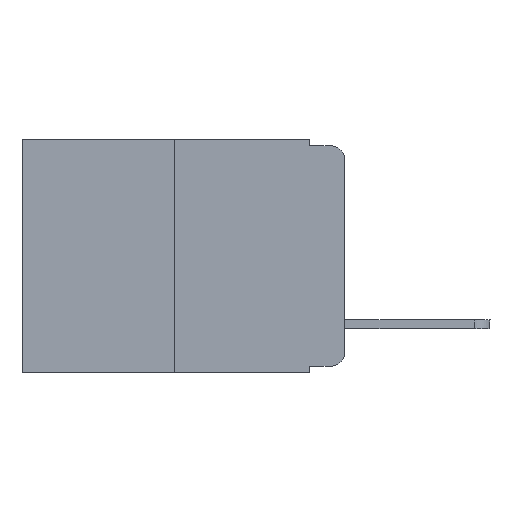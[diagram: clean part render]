
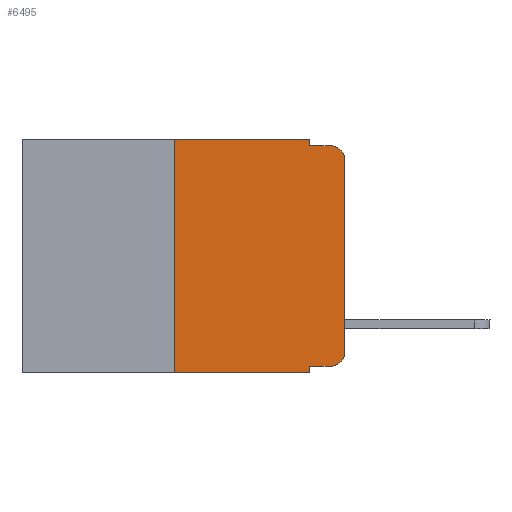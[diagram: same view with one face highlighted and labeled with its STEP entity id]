
A CAD part, left-side view. The second image highlights one B-rep face of the part: STEP entity #6495.
In plain terms, the highlighted planar face has unit normal (-1, 0, 0).
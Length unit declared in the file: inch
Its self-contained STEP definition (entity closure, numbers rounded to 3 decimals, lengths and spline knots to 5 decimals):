
#187 = AXIS2_PLACEMENT_3D ( 'NONE', #8793, #5177, #2572 ) ;
#358 = LINE ( 'NONE', #3914, #7041 ) ;
#514 = VECTOR ( 'NONE', #11091, 39.37008 ) ;
#615 = CARTESIAN_POINT ( 'NONE',  ( 0., 0.051, -0.333 ) ) ;
#802 = CARTESIAN_POINT ( 'NONE',  ( 0., 0.02, -0.01 ) ) ;
#941 = VECTOR ( 'NONE', #5266, 39.37008 ) ;
#1002 = CARTESIAN_POINT ( 'NONE',  ( 0., 0.473, -0.343 ) ) ;
#1118 = LINE ( 'NONE', #1002, #8126 ) ;
#1142 = VERTEX_POINT ( 'NONE', #10294 ) ;
#1150 = CIRCLE ( 'NONE', #4864, 0.02 ) ;
#1329 = FACE_OUTER_BOUND ( 'NONE', #9401, .T. ) ;
#1379 = CARTESIAN_POINT ( 'NONE',  ( 0., 0.02, -0.313 ) ) ;
#1522 = VERTEX_POINT ( 'NONE', #4796 ) ;
#1775 = CARTESIAN_POINT ( 'NONE',  ( 0., 0.25, 0. ) ) ;
#2172 = VECTOR ( 'NONE', #7994, 39.37008 ) ;
#2470 = ORIENTED_EDGE ( 'NONE', *, *, #10821, .F. ) ;
#2572 = DIRECTION ( 'NONE',  ( 0., 0., -1. ) ) ;
#2610 = CARTESIAN_POINT ( 'NONE',  ( 0., 0.473, 0. ) ) ;
#2614 = EDGE_CURVE ( 'NONE', #10281, #10772, #10643, .T. ) ;
#2779 = VECTOR ( 'NONE', #10279, 39.37008 ) ;
#2818 = DIRECTION ( 'NONE',  ( 0., -1., 0. ) ) ;
#2847 = VERTEX_POINT ( 'NONE', #8416 ) ;
#2932 = EDGE_CURVE ( 'NONE', #11075, #1522, #4972, .T. ) ;
#3179 = CARTESIAN_POINT ( 'NONE',  ( 0., 0.051, 0. ) ) ;
#3510 = ORIENTED_EDGE ( 'NONE', *, *, #5780, .T. ) ;
#3914 = CARTESIAN_POINT ( 'NONE',  ( 0., 0.25, 0. ) ) ;
#4440 = CARTESIAN_POINT ( 'NONE',  ( 0., 0.051, 0. ) ) ;
#4601 = ORIENTED_EDGE ( 'NONE', *, *, #9011, .T. ) ;
#4796 = CARTESIAN_POINT ( 'NONE',  ( 0., 0.02, -0.333 ) ) ;
#4849 = VERTEX_POINT ( 'NONE', #5217 ) ;
#4864 = AXIS2_PLACEMENT_3D ( 'NONE', #1379, #6551, #11170 ) ;
#4945 = AXIS2_PLACEMENT_3D ( 'NONE', #5795, #9243, #5850 ) ;
#4972 = LINE ( 'NONE', #615, #2779 ) ;
#4986 = CIRCLE ( 'NONE', #187, 0.02 ) ;
#5103 = CARTESIAN_POINT ( 'NONE',  ( 0., 0., 0. ) ) ;
#5177 = DIRECTION ( 'NONE',  ( -1., 0., 0. ) ) ;
#5215 = EDGE_CURVE ( 'NONE', #1522, #4849, #1150, .T. ) ;
#5217 = CARTESIAN_POINT ( 'NONE',  ( 0., 0., -0.313 ) ) ;
#5266 = DIRECTION ( 'NONE',  ( 0., -1., 0. ) ) ;
#5332 = DIRECTION ( 'NONE',  ( 0., 0., 1. ) ) ;
#5400 = CARTESIAN_POINT ( 'NONE',  ( 0., 0.051, -0.01 ) ) ;
#5403 = ORIENTED_EDGE ( 'NONE', *, *, #7142, .F. ) ;
#5424 = LINE ( 'NONE', #4440, #2172 ) ;
#5591 = DIRECTION ( 'NONE',  ( 0., -1., 0. ) ) ;
#5780 = EDGE_CURVE ( 'NONE', #1142, #8042, #4986, .T. ) ;
#5795 = CARTESIAN_POINT ( 'NONE',  ( 0., 0.473, 0. ) ) ;
#5850 = DIRECTION ( 'NONE',  ( 0., 0., -1. ) ) ;
#6495 = ADVANCED_FACE ( 'NONE', ( #1329 ), #6503, .F. ) ;
#6503 = PLANE ( 'NONE',  #4945 ) ;
#6551 = DIRECTION ( 'NONE',  ( -1., 0., 0. ) ) ;
#6909 = LINE ( 'NONE', #5103, #9968 ) ;
#7041 = VECTOR ( 'NONE', #7451, 39.37008 ) ;
#7142 = EDGE_CURVE ( 'NONE', #11075, #2847, #5424, .T. ) ;
#7417 = LINE ( 'NONE', #3179, #514 ) ;
#7451 = DIRECTION ( 'NONE',  ( 0., 0., 1. ) ) ;
#7865 = ORIENTED_EDGE ( 'NONE', *, *, #8797, .F. ) ;
#7994 = DIRECTION ( 'NONE',  ( 0., 0., -1. ) ) ;
#8042 = VERTEX_POINT ( 'NONE', #802 ) ;
#8126 = VECTOR ( 'NONE', #2818, 39.37008 ) ;
#8128 = EDGE_CURVE ( 'NONE', #4849, #1142, #6909, .T. ) ;
#8416 = CARTESIAN_POINT ( 'NONE',  ( 0., 0.051, -0.343 ) ) ;
#8437 = CARTESIAN_POINT ( 'NONE',  ( 0., 0.051, -0.01 ) ) ;
#8720 = VECTOR ( 'NONE', #5591, 39.37008 ) ;
#8756 = CARTESIAN_POINT ( 'NONE',  ( 0., 0.25, -0.343 ) ) ;
#8793 = CARTESIAN_POINT ( 'NONE',  ( 0., 0.02, -0.03 ) ) ;
#8797 = EDGE_CURVE ( 'NONE', #10772, #9512, #7417, .T. ) ;
#8831 = ORIENTED_EDGE ( 'NONE', *, *, #8128, .T. ) ;
#8908 = CARTESIAN_POINT ( 'NONE',  ( 0., 0.051, -0.333 ) ) ;
#8967 = ORIENTED_EDGE ( 'NONE', *, *, #2932, .T. ) ;
#9011 = EDGE_CURVE ( 'NONE', #10136, #2847, #1118, .T. ) ;
#9243 = DIRECTION ( 'NONE',  ( 1., 0., 0. ) ) ;
#9401 = EDGE_LOOP ( 'NONE', ( #8831, #3510, #9523, #7865, #10854, #2470, #4601, #5403, #8967, #10077 ) ) ;
#9512 = VERTEX_POINT ( 'NONE', #5400 ) ;
#9523 = ORIENTED_EDGE ( 'NONE', *, *, #10765, .F. ) ;
#9968 = VECTOR ( 'NONE', #5332, 39.37008 ) ;
#10077 = ORIENTED_EDGE ( 'NONE', *, *, #5215, .T. ) ;
#10136 = VERTEX_POINT ( 'NONE', #8756 ) ;
#10279 = DIRECTION ( 'NONE',  ( 0., -1., 0. ) ) ;
#10281 = VERTEX_POINT ( 'NONE', #1775 ) ;
#10294 = CARTESIAN_POINT ( 'NONE',  ( 0., 0., -0.03 ) ) ;
#10643 = LINE ( 'NONE', #2610, #941 ) ;
#10680 = CARTESIAN_POINT ( 'NONE',  ( 0., 0.051, 0. ) ) ;
#10765 = EDGE_CURVE ( 'NONE', #9512, #8042, #10897, .T. ) ;
#10772 = VERTEX_POINT ( 'NONE', #10680 ) ;
#10821 = EDGE_CURVE ( 'NONE', #10136, #10281, #358, .T. ) ;
#10854 = ORIENTED_EDGE ( 'NONE', *, *, #2614, .F. ) ;
#10897 = LINE ( 'NONE', #8437, #8720 ) ;
#11075 = VERTEX_POINT ( 'NONE', #8908 ) ;
#11091 = DIRECTION ( 'NONE',  ( 0., 0., -1. ) ) ;
#11170 = DIRECTION ( 'NONE',  ( 0., 0., -1. ) ) ;
